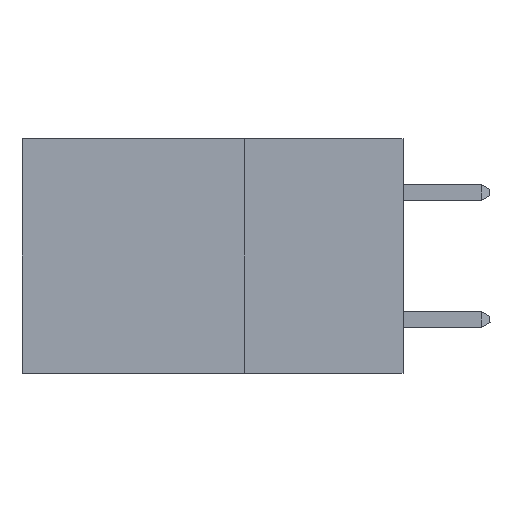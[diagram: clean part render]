
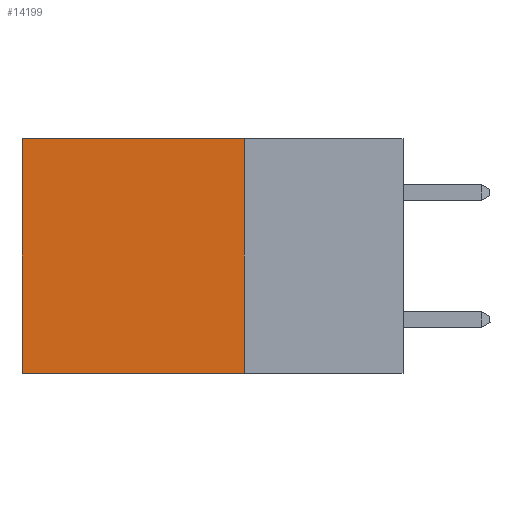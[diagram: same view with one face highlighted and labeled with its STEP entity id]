
A CAD part, left-side view. The second image highlights one B-rep face of the part: STEP entity #14199.
In plain terms, the highlighted planar face has unit normal (-1, 0, 0).
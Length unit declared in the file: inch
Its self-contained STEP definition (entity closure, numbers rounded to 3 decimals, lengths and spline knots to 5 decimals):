
#293 = CARTESIAN_POINT ( 'NONE',  ( 0.2875, 0.6, -0.37 ) ) ;
#596 = LINE ( 'NONE', #14635, #2503 ) ;
#701 = DIRECTION ( 'NONE',  ( 0., 1., 0. ) ) ;
#772 = CARTESIAN_POINT ( 'NONE',  ( 0.2875, 0.25, -0.37 ) ) ;
#1673 = DIRECTION ( 'NONE',  ( 0., 0., -1. ) ) ;
#1697 = LINE ( 'NONE', #772, #12610 ) ;
#2091 = CARTESIAN_POINT ( 'NONE',  ( 0.2875, 0.25, 0. ) ) ;
#2098 = LINE ( 'NONE', #6110, #10220 ) ;
#2503 = VECTOR ( 'NONE', #1673, 39.37008 ) ;
#3083 = EDGE_CURVE ( 'NONE', #9066, #12467, #596, .T. ) ;
#3255 = CARTESIAN_POINT ( 'NONE',  ( 0.2875, 0.25, -0.37 ) ) ;
#3664 = CARTESIAN_POINT ( 'NONE',  ( 0.2875, 0.25, 0. ) ) ;
#3671 = CARTESIAN_POINT ( 'NONE',  ( 0.2875, 0.6, 0. ) ) ;
#3752 = LINE ( 'NONE', #5374, #5066 ) ;
#3895 = EDGE_CURVE ( 'NONE', #10713, #9066, #3752, .T. ) ;
#3901 = EDGE_LOOP ( 'NONE', ( #4481, #7247, #5770, #8992 ) ) ;
#4209 = VERTEX_POINT ( 'NONE', #3255 ) ;
#4481 = ORIENTED_EDGE ( 'NONE', *, *, #3083, .T. ) ;
#4545 = DIRECTION ( 'NONE',  ( 1., 0., 0. ) ) ;
#5050 = EDGE_CURVE ( 'NONE', #4209, #12467, #1697, .T. ) ;
#5066 = VECTOR ( 'NONE', #701, 39.37008 ) ;
#5374 = CARTESIAN_POINT ( 'NONE',  ( 0.2875, 0.25, 0. ) ) ;
#5595 = DIRECTION ( 'NONE',  ( 0., 1., 0. ) ) ;
#5766 = FACE_OUTER_BOUND ( 'NONE', #3901, .T. ) ;
#5770 = ORIENTED_EDGE ( 'NONE', *, *, #11799, .F. ) ;
#6110 = CARTESIAN_POINT ( 'NONE',  ( 0.2875, 0.25, 0. ) ) ;
#6215 = DIRECTION ( 'NONE',  ( 0., 0., -1. ) ) ;
#7247 = ORIENTED_EDGE ( 'NONE', *, *, #5050, .F. ) ;
#7579 = AXIS2_PLACEMENT_3D ( 'NONE', #2091, #4545, #12637 ) ;
#8992 = ORIENTED_EDGE ( 'NONE', *, *, #3895, .T. ) ;
#9066 = VERTEX_POINT ( 'NONE', #3671 ) ;
#10220 = VECTOR ( 'NONE', #6215, 39.37008 ) ;
#10257 = PLANE ( 'NONE',  #7579 ) ;
#10713 = VERTEX_POINT ( 'NONE', #3664 ) ;
#11799 = EDGE_CURVE ( 'NONE', #10713, #4209, #2098, .T. ) ;
#12467 = VERTEX_POINT ( 'NONE', #293 ) ;
#12610 = VECTOR ( 'NONE', #5595, 39.37008 ) ;
#12637 = DIRECTION ( 'NONE',  ( 0., 0., -1. ) ) ;
#14199 = ADVANCED_FACE ( 'NONE', ( #5766 ), #10257, .F. ) ;
#14635 = CARTESIAN_POINT ( 'NONE',  ( 0.2875, 0.6, 0. ) ) ;
